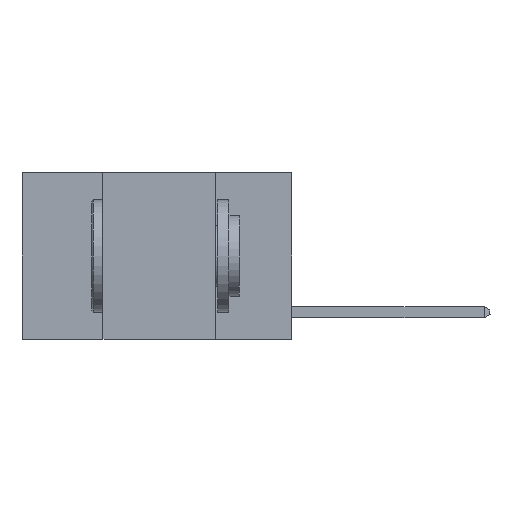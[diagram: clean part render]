
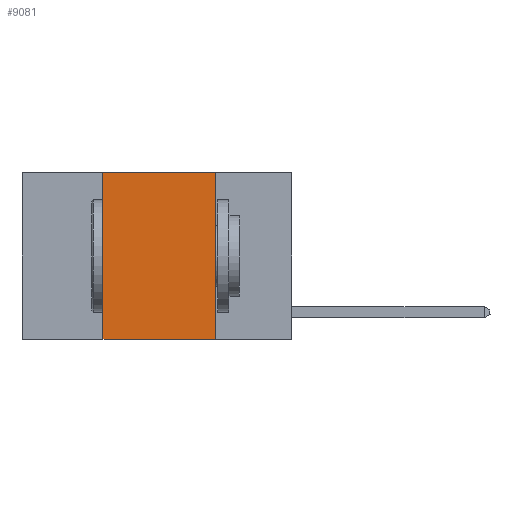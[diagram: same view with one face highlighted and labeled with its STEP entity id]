
A CAD part, left-side view. The second image highlights one B-rep face of the part: STEP entity #9081.
In plain terms, the highlighted planar face has unit normal (-1, 0, 0).
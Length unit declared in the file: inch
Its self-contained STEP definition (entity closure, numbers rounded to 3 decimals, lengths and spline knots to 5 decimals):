
#963 = CARTESIAN_POINT ( 'NONE',  ( 0., 0.6, -0.37 ) ) ;
#994 = VERTEX_POINT ( 'NONE', #10132 ) ;
#1796 = LINE ( 'NONE', #10137, #10554 ) ;
#1859 = LINE ( 'NONE', #11909, #14677 ) ;
#1923 = DIRECTION ( 'NONE',  ( 0., -1., 0. ) ) ;
#2243 = EDGE_CURVE ( 'NONE', #2599, #4938, #1796, .T. ) ;
#2400 = CARTESIAN_POINT ( 'NONE',  ( 0., 0.6, 0. ) ) ;
#2599 = VERTEX_POINT ( 'NONE', #7502 ) ;
#2974 = VECTOR ( 'NONE', #1923, 39.37008 ) ;
#3720 = LINE ( 'NONE', #2400, #12294 ) ;
#4153 = CARTESIAN_POINT ( 'NONE',  ( 0., 0.42, 0. ) ) ;
#4270 = DIRECTION ( 'NONE',  ( 0., 0., -1. ) ) ;
#4415 = VERTEX_POINT ( 'NONE', #13608 ) ;
#4938 = VERTEX_POINT ( 'NONE', #4153 ) ;
#5475 = DIRECTION ( 'NONE',  ( 0., 0., 1. ) ) ;
#5648 = ORIENTED_EDGE ( 'NONE', *, *, #2243, .F. ) ;
#5966 = ORIENTED_EDGE ( 'NONE', *, *, #13900, .F. ) ;
#7122 = DIRECTION ( 'NONE',  ( 0., -1., 0. ) ) ;
#7502 = CARTESIAN_POINT ( 'NONE',  ( 0., 0.42, -0.37 ) ) ;
#7839 = PLANE ( 'NONE',  #13752 ) ;
#7965 = EDGE_LOOP ( 'NONE', ( #15556, #5966, #5648, #14859 ) ) ;
#8005 = DIRECTION ( 'NONE',  ( 1., 0., 0. ) ) ;
#9081 = ADVANCED_FACE ( 'NONE', ( #12744 ), #7839, .F. ) ;
#10132 = CARTESIAN_POINT ( 'NONE',  ( 0., 0.17, -0.37 ) ) ;
#10137 = CARTESIAN_POINT ( 'NONE',  ( 0., 0.42, 0. ) ) ;
#10554 = VECTOR ( 'NONE', #5475, 39.37008 ) ;
#11909 = CARTESIAN_POINT ( 'NONE',  ( 0., 0.17, 0. ) ) ;
#12294 = VECTOR ( 'NONE', #7122, 39.37008 ) ;
#12744 = FACE_OUTER_BOUND ( 'NONE', #7965, .T. ) ;
#13119 = EDGE_CURVE ( 'NONE', #2599, #994, #15722, .T. ) ;
#13608 = CARTESIAN_POINT ( 'NONE',  ( 0., 0.17, 0. ) ) ;
#13752 = AXIS2_PLACEMENT_3D ( 'NONE', #14364, #8005, #4270 ) ;
#13900 = EDGE_CURVE ( 'NONE', #4938, #4415, #3720, .T. ) ;
#14364 = CARTESIAN_POINT ( 'NONE',  ( 0., 0.6, 0. ) ) ;
#14632 = EDGE_CURVE ( 'NONE', #4415, #994, #1859, .T. ) ;
#14677 = VECTOR ( 'NONE', #15405, 39.37008 ) ;
#14859 = ORIENTED_EDGE ( 'NONE', *, *, #13119, .T. ) ;
#15405 = DIRECTION ( 'NONE',  ( 0., 0., -1. ) ) ;
#15556 = ORIENTED_EDGE ( 'NONE', *, *, #14632, .F. ) ;
#15722 = LINE ( 'NONE', #963, #2974 ) ;
